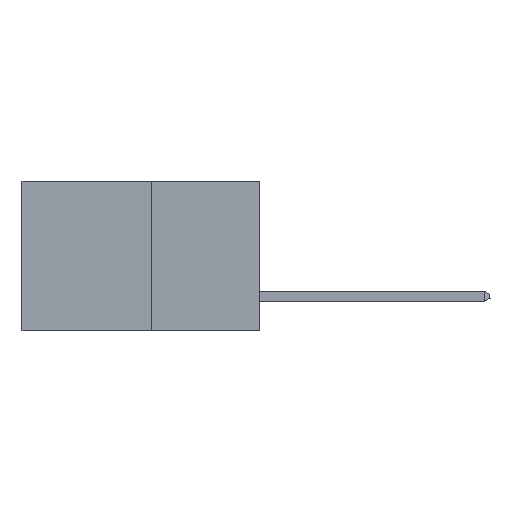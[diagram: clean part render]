
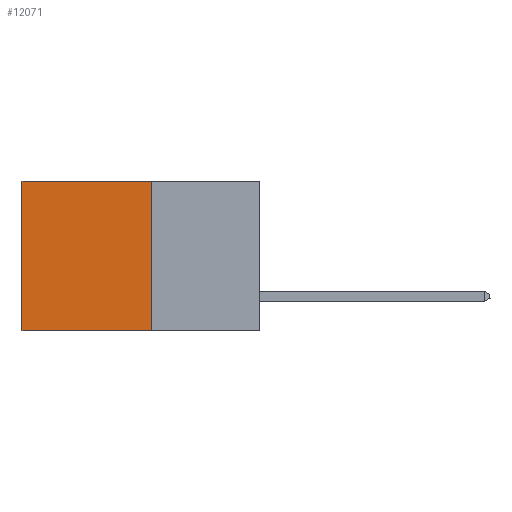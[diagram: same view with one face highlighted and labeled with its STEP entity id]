
A CAD part, left-side view. The second image highlights one B-rep face of the part: STEP entity #12071.
In plain terms, the highlighted planar face has unit normal (-1, 0, 0).
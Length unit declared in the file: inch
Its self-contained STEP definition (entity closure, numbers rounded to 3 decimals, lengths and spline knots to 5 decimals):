
#124 = LINE ( 'NONE', #16797, #7773 ) ;
#295 = CARTESIAN_POINT ( 'NONE',  ( 0.277, 0.27, 0. ) ) ;
#407 = VERTEX_POINT ( 'NONE', #12708 ) ;
#1149 = EDGE_CURVE ( 'NONE', #3642, #17826, #19813, .T. ) ;
#1189 = DIRECTION ( 'NONE',  ( 0., 0., -1. ) ) ;
#2662 = VECTOR ( 'NONE', #11002, 39.37008 ) ;
#3642 = VERTEX_POINT ( 'NONE', #11266 ) ;
#3755 = EDGE_LOOP ( 'NONE', ( #6982, #4262, #18221, #17506 ) ) ;
#4168 = AXIS2_PLACEMENT_3D ( 'NONE', #14945, #5636, #16503 ) ;
#4262 = ORIENTED_EDGE ( 'NONE', *, *, #17515, .F. ) ;
#5636 = DIRECTION ( 'NONE',  ( 1., 0., 0. ) ) ;
#5773 = LINE ( 'NONE', #18424, #17689 ) ;
#6226 = LINE ( 'NONE', #295, #2662 ) ;
#6982 = ORIENTED_EDGE ( 'NONE', *, *, #11580, .T. ) ;
#7439 = CARTESIAN_POINT ( 'NONE',  ( 0.277, 0.59, -0.37 ) ) ;
#7503 = VECTOR ( 'NONE', #1189, 39.37008 ) ;
#7773 = VECTOR ( 'NONE', #18326, 39.37008 ) ;
#10221 = PLANE ( 'NONE',  #4168 ) ;
#10622 = DIRECTION ( 'NONE',  ( 0., 1., 0. ) ) ;
#11002 = DIRECTION ( 'NONE',  ( 0., 1., 0. ) ) ;
#11266 = CARTESIAN_POINT ( 'NONE',  ( 0.277, 0.27, 0. ) ) ;
#11580 = EDGE_CURVE ( 'NONE', #407, #14135, #124, .T. ) ;
#12071 = ADVANCED_FACE ( 'NONE', ( #15038 ), #10221, .F. ) ;
#12708 = CARTESIAN_POINT ( 'NONE',  ( 0.277, 0.59, 0. ) ) ;
#14135 = VERTEX_POINT ( 'NONE', #7439 ) ;
#14945 = CARTESIAN_POINT ( 'NONE',  ( 0.277, 0.27, -0.37 ) ) ;
#15038 = FACE_OUTER_BOUND ( 'NONE', #3755, .T. ) ;
#16503 = DIRECTION ( 'NONE',  ( 0., 0., -1. ) ) ;
#16797 = CARTESIAN_POINT ( 'NONE',  ( 0.277, 0.59, -0.37 ) ) ;
#17462 = CARTESIAN_POINT ( 'NONE',  ( 0.277, 0.27, -0.37 ) ) ;
#17506 = ORIENTED_EDGE ( 'NONE', *, *, #18281, .T. ) ;
#17515 = EDGE_CURVE ( 'NONE', #17826, #14135, #5773, .T. ) ;
#17689 = VECTOR ( 'NONE', #10622, 39.37008 ) ;
#17826 = VERTEX_POINT ( 'NONE', #19135 ) ;
#18221 = ORIENTED_EDGE ( 'NONE', *, *, #1149, .F. ) ;
#18281 = EDGE_CURVE ( 'NONE', #3642, #407, #6226, .T. ) ;
#18326 = DIRECTION ( 'NONE',  ( 0., 0., -1. ) ) ;
#18424 = CARTESIAN_POINT ( 'NONE',  ( 0.277, 0.27, -0.37 ) ) ;
#19135 = CARTESIAN_POINT ( 'NONE',  ( 0.277, 0.27, -0.37 ) ) ;
#19813 = LINE ( 'NONE', #17462, #7503 ) ;
